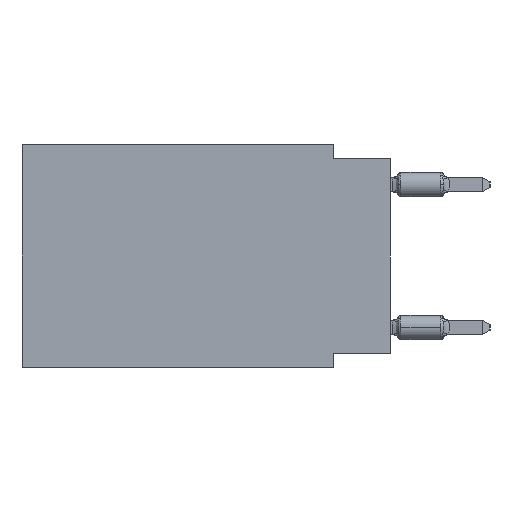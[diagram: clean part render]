
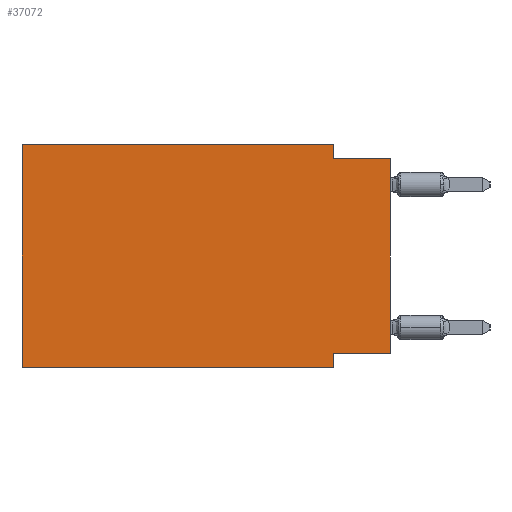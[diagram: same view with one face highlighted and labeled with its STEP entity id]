
A CAD part, left-side view. The second image highlights one B-rep face of the part: STEP entity #37072.
In plain terms, the highlighted planar face has unit normal (-1, 0, 0).
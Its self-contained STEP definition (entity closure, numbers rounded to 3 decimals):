
#436 = VECTOR ( 'NONE', #33623, 1000. ) ;
#2622 = EDGE_LOOP ( 'NONE', ( #31794, #39757, #8911, #14854, #7344, #20476, #37287, #43959 ) ) ;
#3334 = EDGE_CURVE ( 'NONE', #12759, #47260, #16798, .T. ) ;
#3404 = VERTEX_POINT ( 'NONE', #14525 ) ;
#3981 = CARTESIAN_POINT ( 'NONE',  ( 0., 2.54, -9.271 ) ) ;
#4784 = CARTESIAN_POINT ( 'NONE',  ( 0., 2.54, -0.635 ) ) ;
#5435 = PLANE ( 'NONE',  #37916 ) ;
#6387 = EDGE_CURVE ( 'NONE', #3404, #33194, #46324, .T. ) ;
#6505 = VECTOR ( 'NONE', #42315, 1000. ) ;
#6699 = CARTESIAN_POINT ( 'NONE',  ( 0., 0., 0. ) ) ;
#7344 = ORIENTED_EDGE ( 'NONE', *, *, #29719, .F. ) ;
#8911 = ORIENTED_EDGE ( 'NONE', *, *, #19080, .F. ) ;
#12746 = CARTESIAN_POINT ( 'NONE',  ( 0., 0., -0.635 ) ) ;
#12759 = VERTEX_POINT ( 'NONE', #4784 ) ;
#12789 = CARTESIAN_POINT ( 'NONE',  ( 0., 0., -0.635 ) ) ;
#13659 = CARTESIAN_POINT ( 'NONE',  ( 0., 2.54, 0. ) ) ;
#13971 = CARTESIAN_POINT ( 'NONE',  ( 0., 16.383, 0. ) ) ;
#14525 = CARTESIAN_POINT ( 'NONE',  ( 0., 16.383, 0. ) ) ;
#14854 = ORIENTED_EDGE ( 'NONE', *, *, #6387, .F. ) ;
#16301 = EDGE_CURVE ( 'NONE', #23250, #47260, #23005, .T. ) ;
#16798 = LINE ( 'NONE', #12789, #24061 ) ;
#17474 = FACE_OUTER_BOUND ( 'NONE', #2622, .T. ) ;
#18229 = DIRECTION ( 'NONE',  ( 0., 0., 1. ) ) ;
#18317 = CARTESIAN_POINT ( 'NONE',  ( 0., 2.54, -9.906 ) ) ;
#18541 = DIRECTION ( 'NONE',  ( 0., 0., -1. ) ) ;
#19080 = EDGE_CURVE ( 'NONE', #33194, #12759, #41878, .T. ) ;
#19288 = LINE ( 'NONE', #22063, #26110 ) ;
#20476 = ORIENTED_EDGE ( 'NONE', *, *, #36780, .T. ) ;
#21118 = CARTESIAN_POINT ( 'NONE',  ( 0., 0., -9.271 ) ) ;
#22063 = CARTESIAN_POINT ( 'NONE',  ( 0., 16.383, 0. ) ) ;
#22400 = EDGE_CURVE ( 'NONE', #23250, #29697, #23694, .T. ) ;
#23005 = LINE ( 'NONE', #6699, #46328 ) ;
#23250 = VERTEX_POINT ( 'NONE', #21118 ) ;
#23466 = VECTOR ( 'NONE', #24848, 1000. ) ;
#23694 = LINE ( 'NONE', #24178, #26406 ) ;
#24061 = VECTOR ( 'NONE', #32093, 1000. ) ;
#24178 = CARTESIAN_POINT ( 'NONE',  ( 0., 0., -9.271 ) ) ;
#24848 = DIRECTION ( 'NONE',  ( 0., -1., 0. ) ) ;
#26110 = VECTOR ( 'NONE', #33842, 1000. ) ;
#26406 = VECTOR ( 'NONE', #43225, 1000. ) ;
#26837 = CARTESIAN_POINT ( 'NONE',  ( 0., 2.54, 0. ) ) ;
#28387 = VERTEX_POINT ( 'NONE', #38028 ) ;
#29285 = DIRECTION ( 'NONE',  ( 1., 0., 0. ) ) ;
#29697 = VERTEX_POINT ( 'NONE', #3981 ) ;
#29719 = EDGE_CURVE ( 'NONE', #28387, #3404, #19288, .T. ) ;
#30368 = VERTEX_POINT ( 'NONE', #37173 ) ;
#31794 = ORIENTED_EDGE ( 'NONE', *, *, #16301, .T. ) ;
#32093 = DIRECTION ( 'NONE',  ( 0., -1., 0. ) ) ;
#33194 = VERTEX_POINT ( 'NONE', #13659 ) ;
#33623 = DIRECTION ( 'NONE',  ( 0., 0., -1. ) ) ;
#33842 = DIRECTION ( 'NONE',  ( 0., 0., 1. ) ) ;
#34129 = LINE ( 'NONE', #18317, #436 ) ;
#34326 = CARTESIAN_POINT ( 'NONE',  ( 0., 16.383, -9.906 ) ) ;
#35263 = CARTESIAN_POINT ( 'NONE',  ( 0., 16.383, 0. ) ) ;
#35272 = VECTOR ( 'NONE', #18541, 1000. ) ;
#36780 = EDGE_CURVE ( 'NONE', #28387, #30368, #38093, .T. ) ;
#37072 = ADVANCED_FACE ( 'NONE', ( #17474 ), #5435, .F. ) ;
#37173 = CARTESIAN_POINT ( 'NONE',  ( 0., 2.54, -9.906 ) ) ;
#37287 = ORIENTED_EDGE ( 'NONE', *, *, #40113, .F. ) ;
#37916 = AXIS2_PLACEMENT_3D ( 'NONE', #13971, #29285, #44577 ) ;
#38028 = CARTESIAN_POINT ( 'NONE',  ( 0., 16.383, -9.906 ) ) ;
#38093 = LINE ( 'NONE', #34326, #23466 ) ;
#39757 = ORIENTED_EDGE ( 'NONE', *, *, #3334, .F. ) ;
#40113 = EDGE_CURVE ( 'NONE', #29697, #30368, #34129, .T. ) ;
#41878 = LINE ( 'NONE', #26837, #35272 ) ;
#42315 = DIRECTION ( 'NONE',  ( 0., -1., 0. ) ) ;
#43225 = DIRECTION ( 'NONE',  ( 0., 1., 0. ) ) ;
#43959 = ORIENTED_EDGE ( 'NONE', *, *, #22400, .F. ) ;
#44577 = DIRECTION ( 'NONE',  ( 0., 0., -1. ) ) ;
#46324 = LINE ( 'NONE', #35263, #6505 ) ;
#46328 = VECTOR ( 'NONE', #18229, 1000. ) ;
#47260 = VERTEX_POINT ( 'NONE', #12746 ) ;
